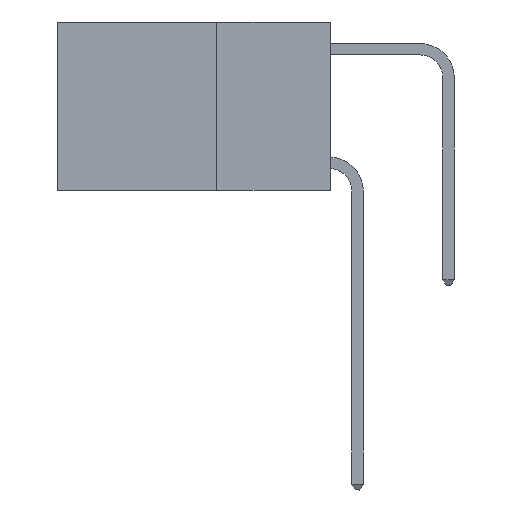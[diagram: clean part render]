
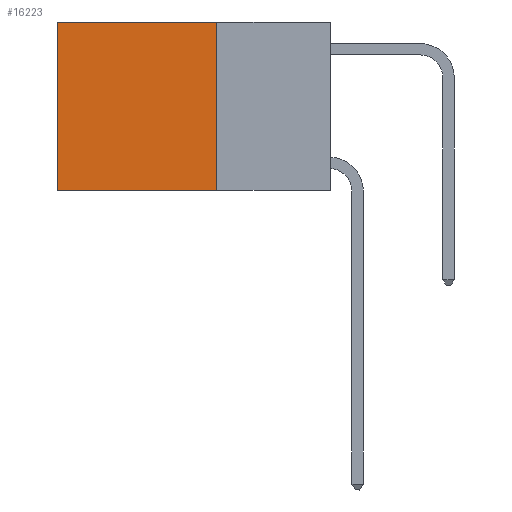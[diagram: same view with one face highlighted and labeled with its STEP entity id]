
A CAD part, left-side view. The second image highlights one B-rep face of the part: STEP entity #16223.
In plain terms, the highlighted planar face has unit normal (-1, 0, 0).
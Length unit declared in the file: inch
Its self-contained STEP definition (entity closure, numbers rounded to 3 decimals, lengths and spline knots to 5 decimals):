
#5 = DIRECTION ( 'NONE',  ( 0., 0., -1. ) ) ;
#1394 = VERTEX_POINT ( 'NONE', #25532 ) ;
#1876 = ORIENTED_EDGE ( 'NONE', *, *, #21552, .F. ) ;
#1891 = ORIENTED_EDGE ( 'NONE', *, *, #5866, .T. ) ;
#1963 = VECTOR ( 'NONE', #7917, 39.37008 ) ;
#2329 = EDGE_LOOP ( 'NONE', ( #20422, #20899, #1876, #1891 ) ) ;
#4347 = PLANE ( 'NONE',  #8655 ) ;
#4407 = CARTESIAN_POINT ( 'NONE',  ( 0.2625, 0.25, 0. ) ) ;
#5866 = EDGE_CURVE ( 'NONE', #1394, #7484, #20901, .T. ) ;
#7484 = VERTEX_POINT ( 'NONE', #25880 ) ;
#7917 = DIRECTION ( 'NONE',  ( 0., 0., -1. ) ) ;
#8438 = EDGE_CURVE ( 'NONE', #17882, #24755, #24152, .T. ) ;
#8655 = AXIS2_PLACEMENT_3D ( 'NONE', #20861, #10484, #5 ) ;
#8722 = FACE_OUTER_BOUND ( 'NONE', #2329, .T. ) ;
#10484 = DIRECTION ( 'NONE',  ( 1., 0., 0. ) ) ;
#11442 = CARTESIAN_POINT ( 'NONE',  ( 0.2625, 0.25, -0.37 ) ) ;
#11812 = LINE ( 'NONE', #22370, #1963 ) ;
#15850 = VECTOR ( 'NONE', #25827, 39.37008 ) ;
#16185 = LINE ( 'NONE', #19692, #15850 ) ;
#16223 = ADVANCED_FACE ( 'NONE', ( #8722 ), #4347, .F. ) ;
#17652 = VECTOR ( 'NONE', #23304, 39.37008 ) ;
#17882 = VERTEX_POINT ( 'NONE', #11442 ) ;
#19223 = EDGE_CURVE ( 'NONE', #7484, #24755, #16185, .T. ) ;
#19692 = CARTESIAN_POINT ( 'NONE',  ( 0.2625, 0.6, 0. ) ) ;
#20422 = ORIENTED_EDGE ( 'NONE', *, *, #19223, .T. ) ;
#20515 = VECTOR ( 'NONE', #27120, 39.37008 ) ;
#20861 = CARTESIAN_POINT ( 'NONE',  ( 0.2625, 0.25, 0. ) ) ;
#20899 = ORIENTED_EDGE ( 'NONE', *, *, #8438, .F. ) ;
#20901 = LINE ( 'NONE', #4407, #17652 ) ;
#21552 = EDGE_CURVE ( 'NONE', #1394, #17882, #11812, .T. ) ;
#22370 = CARTESIAN_POINT ( 'NONE',  ( 0.2625, 0.25, 0. ) ) ;
#23304 = DIRECTION ( 'NONE',  ( 0., 1., 0. ) ) ;
#23525 = CARTESIAN_POINT ( 'NONE',  ( 0.2625, 0.6, -0.37 ) ) ;
#24152 = LINE ( 'NONE', #24762, #20515 ) ;
#24755 = VERTEX_POINT ( 'NONE', #23525 ) ;
#24762 = CARTESIAN_POINT ( 'NONE',  ( 0.2625, 0.25, -0.37 ) ) ;
#25532 = CARTESIAN_POINT ( 'NONE',  ( 0.2625, 0.25, 0. ) ) ;
#25827 = DIRECTION ( 'NONE',  ( 0., 0., -1. ) ) ;
#25880 = CARTESIAN_POINT ( 'NONE',  ( 0.2625, 0.6, 0. ) ) ;
#27120 = DIRECTION ( 'NONE',  ( 0., 1., 0. ) ) ;
